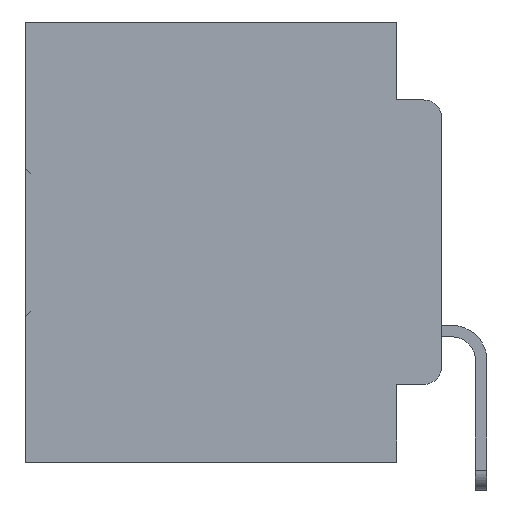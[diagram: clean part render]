
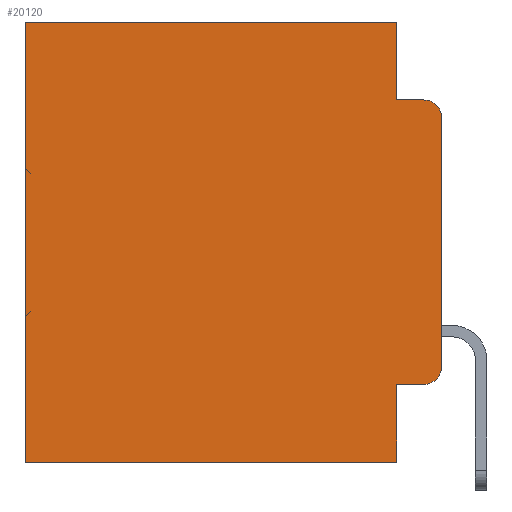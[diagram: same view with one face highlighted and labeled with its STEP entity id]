
A CAD part, left-side view. The second image highlights one B-rep face of the part: STEP entity #20120.
In plain terms, the highlighted planar face has unit normal (-1, 0, 0).
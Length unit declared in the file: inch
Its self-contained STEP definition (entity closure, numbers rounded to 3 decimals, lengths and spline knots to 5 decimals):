
#177 = CARTESIAN_POINT ( 'NONE',  ( 0.298, 0.051, 0. ) ) ;
#1053 = CARTESIAN_POINT ( 'NONE',  ( 0.298, 0.051, 0. ) ) ;
#1437 = CARTESIAN_POINT ( 'NONE',  ( 0.298, 0.473, 0. ) ) ;
#1594 = AXIS2_PLACEMENT_3D ( 'NONE', #19474, #23619, #23822 ) ;
#1744 = CARTESIAN_POINT ( 'NONE',  ( 0.298, 0.473, 0. ) ) ;
#1936 = VERTEX_POINT ( 'NONE', #32251 ) ;
#3025 = DIRECTION ( 'NONE',  ( 0., 0., -1. ) ) ;
#3559 = ORIENTED_EDGE ( 'NONE', *, *, #13646, .F. ) ;
#3643 = CARTESIAN_POINT ( 'NONE',  ( 0.298, 0., 0. ) ) ;
#4221 = CARTESIAN_POINT ( 'NONE',  ( 0.298, 0.051, -0.0885 ) ) ;
#4462 = VECTOR ( 'NONE', #6346, 39.37008 ) ;
#4782 = CARTESIAN_POINT ( 'NONE',  ( 0.298, 0.051, -0.4115 ) ) ;
#5177 = VECTOR ( 'NONE', #9937, 39.37008 ) ;
#5243 = VECTOR ( 'NONE', #3025, 39.37008 ) ;
#6346 = DIRECTION ( 'NONE',  ( 0., -1., 0. ) ) ;
#6363 = EDGE_CURVE ( 'NONE', #13096, #21171, #17579, .T. ) ;
#6634 = LINE ( 'NONE', #1053, #12213 ) ;
#6843 = VECTOR ( 'NONE', #22685, 39.37008 ) ;
#7236 = VERTEX_POINT ( 'NONE', #10441 ) ;
#7603 = DIRECTION ( 'NONE',  ( 0., -1., 0. ) ) ;
#7611 = EDGE_CURVE ( 'NONE', #16030, #31840, #12471, .T. ) ;
#8127 = ORIENTED_EDGE ( 'NONE', *, *, #14095, .F. ) ;
#8448 = CARTESIAN_POINT ( 'NONE',  ( 0.298, 0., 0. ) ) ;
#9105 = CARTESIAN_POINT ( 'NONE',  ( 0.298, 0.051, -0.0885 ) ) ;
#9432 = AXIS2_PLACEMENT_3D ( 'NONE', #12443, #30991, #15152 ) ;
#9487 = EDGE_CURVE ( 'NONE', #7236, #1936, #33222, .T. ) ;
#9532 = VERTEX_POINT ( 'NONE', #4221 ) ;
#9721 = VERTEX_POINT ( 'NONE', #16091 ) ;
#9937 = DIRECTION ( 'NONE',  ( 0., 1., 0. ) ) ;
#10157 = FACE_OUTER_BOUND ( 'NONE', #24925, .T. ) ;
#10441 = CARTESIAN_POINT ( 'NONE',  ( 0.298, 0.02, -0.4115 ) ) ;
#10467 = VECTOR ( 'NONE', #7603, 39.37008 ) ;
#10497 = ORIENTED_EDGE ( 'NONE', *, *, #9487, .T. ) ;
#11316 = PLANE ( 'NONE',  #34957 ) ;
#12213 = VECTOR ( 'NONE', #14847, 39.37008 ) ;
#12443 = CARTESIAN_POINT ( 'NONE',  ( 0.298, 0.02, -0.3915 ) ) ;
#12471 = LINE ( 'NONE', #28600, #5177 ) ;
#12778 = CARTESIAN_POINT ( 'NONE',  ( 0.298, 0.051, -0.5 ) ) ;
#13096 = VERTEX_POINT ( 'NONE', #15242 ) ;
#13646 = EDGE_CURVE ( 'NONE', #9721, #29690, #6634, .T. ) ;
#14059 = DIRECTION ( 'NONE',  ( 0., 0., -1. ) ) ;
#14095 = EDGE_CURVE ( 'NONE', #9532, #21171, #32937, .T. ) ;
#14847 = DIRECTION ( 'NONE',  ( 0., 0., -1. ) ) ;
#15152 = DIRECTION ( 'NONE',  ( 0., 0., -1. ) ) ;
#15242 = CARTESIAN_POINT ( 'NONE',  ( 0.298, 0., -0.1085 ) ) ;
#16030 = VERTEX_POINT ( 'NONE', #31161 ) ;
#16091 = CARTESIAN_POINT ( 'NONE',  ( 0.298, 0.051, -0.4115 ) ) ;
#16101 = EDGE_CURVE ( 'NONE', #9721, #7236, #31666, .T. ) ;
#17579 = CIRCLE ( 'NONE', #1594, 0.02 ) ;
#17929 = DIRECTION ( 'NONE',  ( 0., 0., -1. ) ) ;
#18473 = EDGE_CURVE ( 'NONE', #13096, #1936, #21277, .T. ) ;
#18905 = DIRECTION ( 'NONE',  ( 0., 1., 0. ) ) ;
#19474 = CARTESIAN_POINT ( 'NONE',  ( 0.298, 0.02, -0.1085 ) ) ;
#19792 = LINE ( 'NONE', #34657, #26853 ) ;
#20010 = CARTESIAN_POINT ( 'NONE',  ( 0.298, 0.02, -0.0885 ) ) ;
#20120 = ADVANCED_FACE ( 'NONE', ( #10157 ), #11316, .F. ) ;
#20240 = ORIENTED_EDGE ( 'NONE', *, *, #7611, .T. ) ;
#21080 = ORIENTED_EDGE ( 'NONE', *, *, #22592, .T. ) ;
#21171 = VERTEX_POINT ( 'NONE', #20010 ) ;
#21277 = LINE ( 'NONE', #3643, #6843 ) ;
#21875 = VECTOR ( 'NONE', #17929, 39.37008 ) ;
#22592 = EDGE_CURVE ( 'NONE', #31840, #25438, #28831, .T. ) ;
#22685 = DIRECTION ( 'NONE',  ( 0., 0., -1. ) ) ;
#23551 = ORIENTED_EDGE ( 'NONE', *, *, #16101, .T. ) ;
#23619 = DIRECTION ( 'NONE',  ( -1., 0., 0. ) ) ;
#23731 = EDGE_CURVE ( 'NONE', #16030, #9532, #32819, .T. ) ;
#23822 = DIRECTION ( 'NONE',  ( 0., 0., -1. ) ) ;
#24925 = EDGE_LOOP ( 'NONE', ( #25181, #33471, #8127, #32542, #20240, #21080, #25522, #3559, #23551, #10497 ) ) ;
#25181 = ORIENTED_EDGE ( 'NONE', *, *, #18473, .F. ) ;
#25438 = VERTEX_POINT ( 'NONE', #34633 ) ;
#25522 = ORIENTED_EDGE ( 'NONE', *, *, #29822, .F. ) ;
#26853 = VECTOR ( 'NONE', #18905, 39.37008 ) ;
#28600 = CARTESIAN_POINT ( 'NONE',  ( 0.298, 0., 0. ) ) ;
#28831 = LINE ( 'NONE', #1437, #21875 ) ;
#29690 = VERTEX_POINT ( 'NONE', #12778 ) ;
#29822 = EDGE_CURVE ( 'NONE', #29690, #25438, #19792, .T. ) ;
#29911 = DIRECTION ( 'NONE',  ( 1., 0., 0. ) ) ;
#30991 = DIRECTION ( 'NONE',  ( -1., 0., 0. ) ) ;
#31161 = CARTESIAN_POINT ( 'NONE',  ( 0.298, 0.051, 0. ) ) ;
#31666 = LINE ( 'NONE', #4782, #10467 ) ;
#31840 = VERTEX_POINT ( 'NONE', #1744 ) ;
#32251 = CARTESIAN_POINT ( 'NONE',  ( 0.298, 0., -0.3915 ) ) ;
#32542 = ORIENTED_EDGE ( 'NONE', *, *, #23731, .F. ) ;
#32819 = LINE ( 'NONE', #177, #5243 ) ;
#32937 = LINE ( 'NONE', #9105, #4462 ) ;
#33222 = CIRCLE ( 'NONE', #9432, 0.02 ) ;
#33471 = ORIENTED_EDGE ( 'NONE', *, *, #6363, .T. ) ;
#34633 = CARTESIAN_POINT ( 'NONE',  ( 0.298, 0.473, -0.5 ) ) ;
#34657 = CARTESIAN_POINT ( 'NONE',  ( 0.298, 0., -0.5 ) ) ;
#34957 = AXIS2_PLACEMENT_3D ( 'NONE', #8448, #29911, #14059 ) ;
